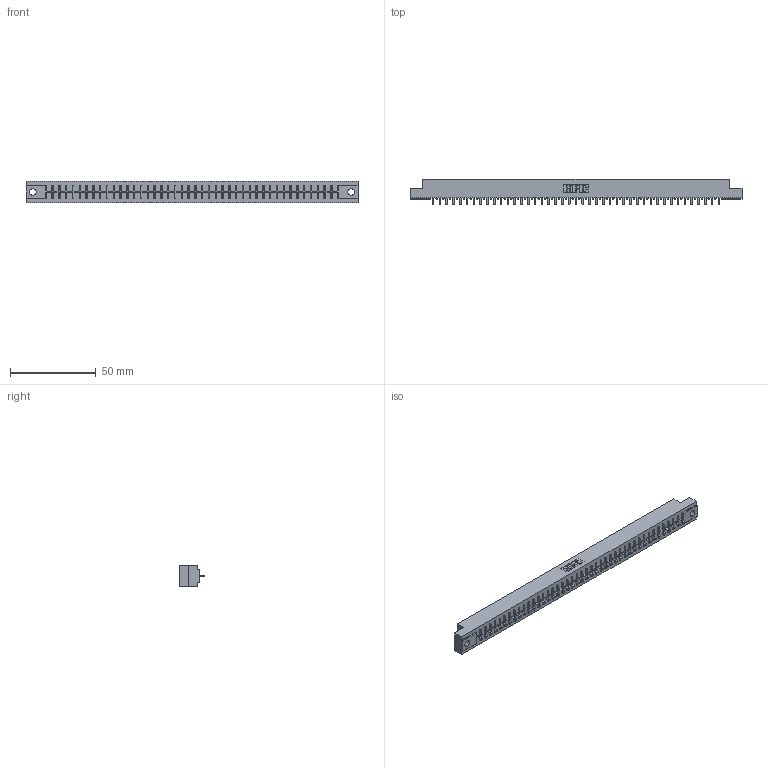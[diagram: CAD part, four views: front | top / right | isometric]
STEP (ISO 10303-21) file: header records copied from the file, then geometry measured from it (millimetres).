
FILE_DESCRIPTION (( 'STEP AP203' ), '1' );
FILE_NAME ('316-043-521-104.STEP', '2018-07-31T06:06:03', ( '' ), ( '' ), 'SwSTEP 2.0', 'SolidWorks 2016', '' );
FILE_SCHEMA (( 'CONFIG_CONTROL_DESIGN' ));
Length unit declared in the file: inch
Products named in the file (3): 306 Part_.156 Dia; 306-290-001_121; 316-043-521-104
Assembly tree (44 placements, depth 2):
  316-043-521-104
    306 Part_.156 Dia
    306-290-001_121  x43
Bounding box: 193.4 x 14.88 x 12.7 mm (x, y, z)
Volume: 21243.8 mm3; surface area: 21306.1 mm2
Topology: 44 solids, 44 shells, 3140 faces, 8823 edges, 5650 vertices
Faces by surface type: plane 2103, cylinder 865, sphere 172
Entity records: 40344 total; most frequent: CARTESIAN_POINT 6778, ORIENTED_EDGE 6718, DIRECTION 6675, EDGE_CURVE 3359, LINE 2637, VECTOR 2637, VERTEX_POINT 2122, AXIS2_PLACEMENT_3D 2019
